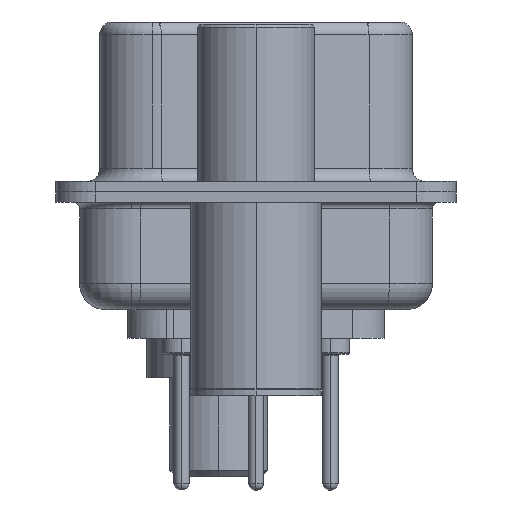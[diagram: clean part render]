
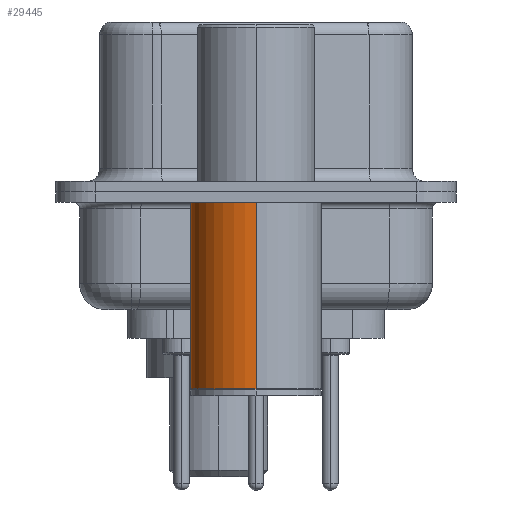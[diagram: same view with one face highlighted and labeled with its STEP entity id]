
A CAD part, left-side view. The second image highlights one B-rep face of the part: STEP entity #29445.
In plain terms, the highlighted cylindrical face has radius 2.5 mm (diameter 5 mm), a partial arc.
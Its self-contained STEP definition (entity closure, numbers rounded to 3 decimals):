
#612 = EDGE_LOOP ( 'NONE', ( #11416, #7101, #24437, #25824 ) ) ;
#959 = AXIS2_PLACEMENT_3D ( 'NONE', #10938, #24787, #13266 ) ;
#2905 = DIRECTION ( 'NONE',  ( 0., 0., 1. ) ) ;
#3714 = CYLINDRICAL_SURFACE ( 'NONE', #959, 2.5 ) ;
#5488 = DIRECTION ( 'NONE',  ( 0., 0., 1. ) ) ;
#5912 = CIRCLE ( 'NONE', #21771, 2.5 ) ;
#6716 = VECTOR ( 'NONE', #18195, 1000. ) ;
#7101 = ORIENTED_EDGE ( 'NONE', *, *, #28927, .T. ) ;
#7840 = CARTESIAN_POINT ( 'NONE',  ( -2.5, 0., 0.581 ) ) ;
#8516 = CARTESIAN_POINT ( 'NONE',  ( 0., 0., -0.4 ) ) ;
#10894 = DIRECTION ( 'NONE',  ( 1., 0., 0. ) ) ;
#10938 = CARTESIAN_POINT ( 'NONE',  ( 0., 0., 0.581 ) ) ;
#11416 = ORIENTED_EDGE ( 'NONE', *, *, #23339, .T. ) ;
#13050 = LINE ( 'NONE', #13531, #6716 ) ;
#13266 = DIRECTION ( 'NONE',  ( 1., 0., 0. ) ) ;
#13323 = CARTESIAN_POINT ( 'NONE',  ( -2.5, 0., -7.525 ) ) ;
#13503 = VERTEX_POINT ( 'NONE', #18486 ) ;
#13531 = CARTESIAN_POINT ( 'NONE',  ( 2.5, 0., 0.581 ) ) ;
#14019 = CARTESIAN_POINT ( 'NONE',  ( 2.5, 0., -7.525 ) ) ;
#15522 = EDGE_CURVE ( 'NONE', #19906, #13503, #5912, .T. ) ;
#17000 = CARTESIAN_POINT ( 'NONE',  ( 0., 0., -7.525 ) ) ;
#17009 = VECTOR ( 'NONE', #5488, 1000. ) ;
#17012 = VERTEX_POINT ( 'NONE', #13323 ) ;
#17703 = FACE_OUTER_BOUND ( 'NONE', #612, .T. ) ;
#17739 = VERTEX_POINT ( 'NONE', #14019 ) ;
#18195 = DIRECTION ( 'NONE',  ( 0., 0., 1. ) ) ;
#18486 = CARTESIAN_POINT ( 'NONE',  ( -2.5, 0., -0.4 ) ) ;
#19293 = DIRECTION ( 'NONE',  ( 1., 0., 0. ) ) ;
#19906 = VERTEX_POINT ( 'NONE', #30008 ) ;
#21771 = AXIS2_PLACEMENT_3D ( 'NONE', #8516, #24747, #10894 ) ;
#23339 = EDGE_CURVE ( 'NONE', #17739, #17012, #23363, .T. ) ;
#23363 = CIRCLE ( 'NONE', #25951, 2.5 ) ;
#24437 = ORIENTED_EDGE ( 'NONE', *, *, #15522, .F. ) ;
#24488 = LINE ( 'NONE', #7840, #17009 ) ;
#24747 = DIRECTION ( 'NONE',  ( 0., 0., 1. ) ) ;
#24787 = DIRECTION ( 'NONE',  ( 0., 0., 1. ) ) ;
#25824 = ORIENTED_EDGE ( 'NONE', *, *, #27769, .F. ) ;
#25951 = AXIS2_PLACEMENT_3D ( 'NONE', #17000, #2905, #19293 ) ;
#27769 = EDGE_CURVE ( 'NONE', #17739, #19906, #13050, .T. ) ;
#28927 = EDGE_CURVE ( 'NONE', #17012, #13503, #24488, .T. ) ;
#29445 = ADVANCED_FACE ( 'NONE', ( #17703 ), #3714, .T. ) ;
#30008 = CARTESIAN_POINT ( 'NONE',  ( 2.5, 0., -0.4 ) ) ;
